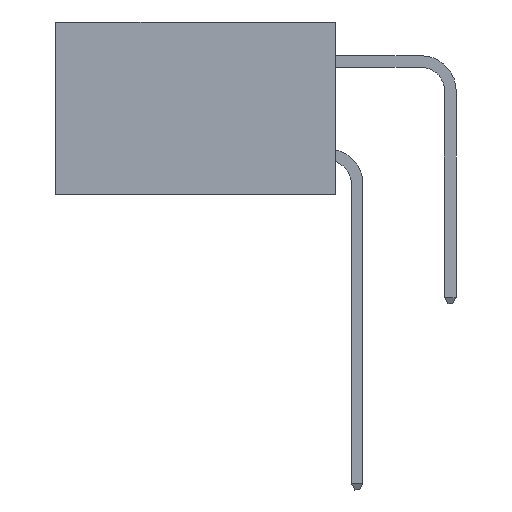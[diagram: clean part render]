
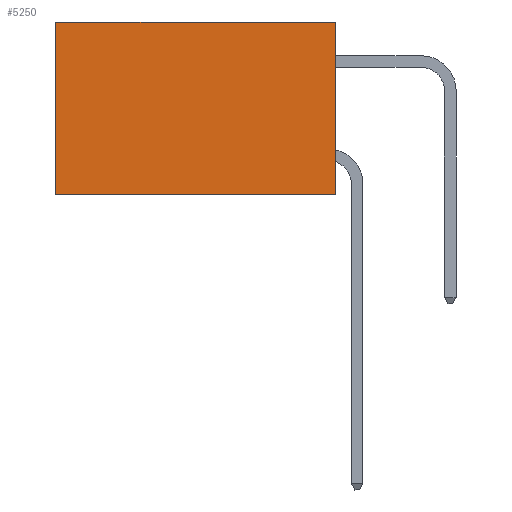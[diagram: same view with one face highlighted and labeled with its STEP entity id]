
A CAD part, left-side view. The second image highlights one B-rep face of the part: STEP entity #5250.
In plain terms, the highlighted planar face has unit normal (-1, 0, 0).
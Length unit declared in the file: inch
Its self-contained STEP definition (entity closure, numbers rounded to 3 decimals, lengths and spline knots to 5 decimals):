
#312 = ORIENTED_EDGE ( 'NONE', *, *, #6770, .F. ) ;
#863 = DIRECTION ( 'NONE',  ( 0., 0., -1. ) ) ;
#939 = LINE ( 'NONE', #1765, #3265 ) ;
#1080 = VERTEX_POINT ( 'NONE', #10170 ) ;
#1558 = ORIENTED_EDGE ( 'NONE', *, *, #10699, .F. ) ;
#1765 = CARTESIAN_POINT ( 'NONE',  ( 0.2875, 0., 0. ) ) ;
#2214 = CARTESIAN_POINT ( 'NONE',  ( 0.2875, 0., 0. ) ) ;
#2761 = DIRECTION ( 'NONE',  ( 0., 1., 0. ) ) ;
#2823 = LINE ( 'NONE', #11783, #5126 ) ;
#3265 = VECTOR ( 'NONE', #2761, 39.37008 ) ;
#3268 = ORIENTED_EDGE ( 'NONE', *, *, #10475, .T. ) ;
#3324 = FACE_OUTER_BOUND ( 'NONE', #9576, .T. ) ;
#3715 = VERTEX_POINT ( 'NONE', #8780 ) ;
#3817 = LINE ( 'NONE', #12646, #6432 ) ;
#4031 = CARTESIAN_POINT ( 'NONE',  ( 0.2875, 0., 0. ) ) ;
#4134 = VECTOR ( 'NONE', #863, 39.37008 ) ;
#4569 = AXIS2_PLACEMENT_3D ( 'NONE', #2214, #11143, #9150 ) ;
#4763 = VERTEX_POINT ( 'NONE', #6511 ) ;
#5126 = VECTOR ( 'NONE', #5584, 39.37008 ) ;
#5250 = ADVANCED_FACE ( 'NONE', ( #3324 ), #7137, .F. ) ;
#5584 = DIRECTION ( 'NONE',  ( 0., 1., 0. ) ) ;
#5669 = LINE ( 'NONE', #4031, #4134 ) ;
#6432 = VECTOR ( 'NONE', #6710, 39.37008 ) ;
#6511 = CARTESIAN_POINT ( 'NONE',  ( 0.2875, 0., 0. ) ) ;
#6710 = DIRECTION ( 'NONE',  ( 0., 0., -1. ) ) ;
#6770 = EDGE_CURVE ( 'NONE', #3715, #8485, #2823, .T. ) ;
#7137 = PLANE ( 'NONE',  #4569 ) ;
#8485 = VERTEX_POINT ( 'NONE', #10509 ) ;
#8780 = CARTESIAN_POINT ( 'NONE',  ( 0.2875, 0., -0.37 ) ) ;
#9150 = DIRECTION ( 'NONE',  ( 0., 0., -1. ) ) ;
#9576 = EDGE_LOOP ( 'NONE', ( #3268, #312, #1558, #9997 ) ) ;
#9997 = ORIENTED_EDGE ( 'NONE', *, *, #12835, .T. ) ;
#10170 = CARTESIAN_POINT ( 'NONE',  ( 0.2875, 0.6, 0. ) ) ;
#10475 = EDGE_CURVE ( 'NONE', #1080, #8485, #3817, .T. ) ;
#10509 = CARTESIAN_POINT ( 'NONE',  ( 0.2875, 0.6, -0.37 ) ) ;
#10699 = EDGE_CURVE ( 'NONE', #4763, #3715, #5669, .T. ) ;
#11143 = DIRECTION ( 'NONE',  ( 1., 0., 0. ) ) ;
#11783 = CARTESIAN_POINT ( 'NONE',  ( 0.2875, 0., -0.37 ) ) ;
#12646 = CARTESIAN_POINT ( 'NONE',  ( 0.2875, 0.6, 0. ) ) ;
#12835 = EDGE_CURVE ( 'NONE', #4763, #1080, #939, .T. ) ;
